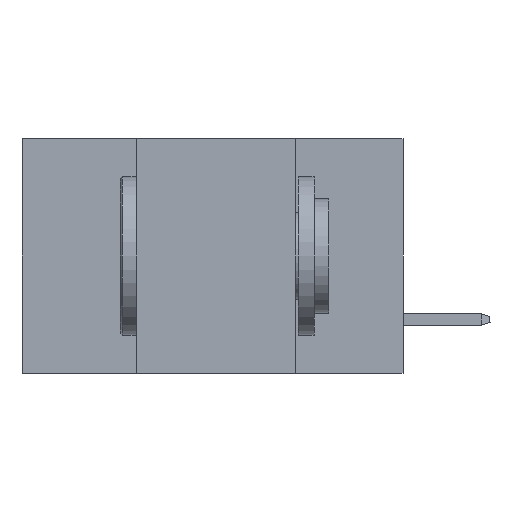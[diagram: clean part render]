
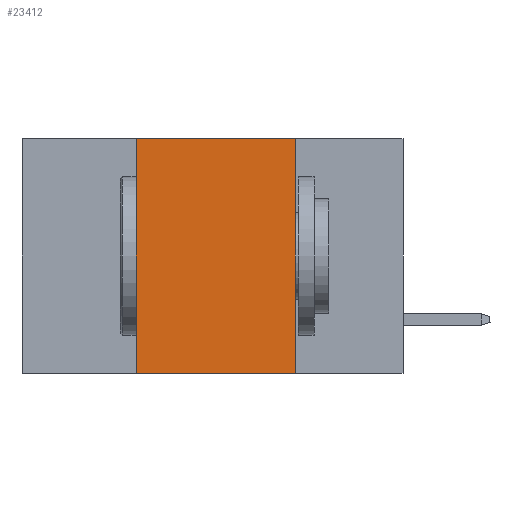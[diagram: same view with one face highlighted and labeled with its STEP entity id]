
A CAD part, left-side view. The second image highlights one B-rep face of the part: STEP entity #23412.
In plain terms, the highlighted planar face has unit normal (-1, 0, 0).
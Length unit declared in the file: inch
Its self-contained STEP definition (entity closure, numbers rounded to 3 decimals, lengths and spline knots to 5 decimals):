
#727 = CARTESIAN_POINT ( 'NONE',  ( 0., 0.17, 0. ) ) ;
#835 = ORIENTED_EDGE ( 'NONE', *, *, #10806, .T. ) ;
#1343 = EDGE_CURVE ( 'NONE', #6513, #32705, #23800, .T. ) ;
#4993 = VECTOR ( 'NONE', #10306, 39.37008 ) ;
#5039 = LINE ( 'NONE', #8041, #4993 ) ;
#6513 = VERTEX_POINT ( 'NONE', #34086 ) ;
#7854 = VERTEX_POINT ( 'NONE', #13912 ) ;
#8041 = CARTESIAN_POINT ( 'NONE',  ( 0., 0.6, -0.37 ) ) ;
#9595 = EDGE_LOOP ( 'NONE', ( #32856, #22056, #18296, #835 ) ) ;
#10010 = AXIS2_PLACEMENT_3D ( 'NONE', #33919, #31629, #19496 ) ;
#10306 = DIRECTION ( 'NONE',  ( 0., -1., 0. ) ) ;
#10806 = EDGE_CURVE ( 'NONE', #16910, #32705, #5039, .T. ) ;
#11239 = EDGE_CURVE ( 'NONE', #7854, #6513, #16242, .T. ) ;
#11932 = VECTOR ( 'NONE', #22219, 39.37008 ) ;
#12795 = LINE ( 'NONE', #31820, #11932 ) ;
#13912 = CARTESIAN_POINT ( 'NONE',  ( 0., 0.42, 0. ) ) ;
#15791 = VECTOR ( 'NONE', #22523, 39.37008 ) ;
#16242 = LINE ( 'NONE', #34087, #15791 ) ;
#16910 = VERTEX_POINT ( 'NONE', #33241 ) ;
#18296 = ORIENTED_EDGE ( 'NONE', *, *, #19326, .F. ) ;
#19326 = EDGE_CURVE ( 'NONE', #16910, #7854, #12795, .T. ) ;
#19496 = DIRECTION ( 'NONE',  ( 0., 0., -1. ) ) ;
#20363 = VECTOR ( 'NONE', #20592, 39.37008 ) ;
#20592 = DIRECTION ( 'NONE',  ( 0., 0., -1. ) ) ;
#21637 = FACE_OUTER_BOUND ( 'NONE', #9595, .T. ) ;
#22056 = ORIENTED_EDGE ( 'NONE', *, *, #11239, .F. ) ;
#22219 = DIRECTION ( 'NONE',  ( 0., 0., 1. ) ) ;
#22523 = DIRECTION ( 'NONE',  ( 0., -1., 0. ) ) ;
#23412 = ADVANCED_FACE ( 'NONE', ( #21637 ), #27502, .F. ) ;
#23800 = LINE ( 'NONE', #727, #20363 ) ;
#24097 = CARTESIAN_POINT ( 'NONE',  ( 0., 0.17, -0.37 ) ) ;
#27502 = PLANE ( 'NONE',  #10010 ) ;
#31629 = DIRECTION ( 'NONE',  ( 1., 0., 0. ) ) ;
#31820 = CARTESIAN_POINT ( 'NONE',  ( 0., 0.42, 0. ) ) ;
#32705 = VERTEX_POINT ( 'NONE', #24097 ) ;
#32856 = ORIENTED_EDGE ( 'NONE', *, *, #1343, .F. ) ;
#33241 = CARTESIAN_POINT ( 'NONE',  ( 0., 0.42, -0.37 ) ) ;
#33919 = CARTESIAN_POINT ( 'NONE',  ( 0., 0.6, 0. ) ) ;
#34086 = CARTESIAN_POINT ( 'NONE',  ( 0., 0.17, 0. ) ) ;
#34087 = CARTESIAN_POINT ( 'NONE',  ( 0., 0.6, 0. ) ) ;
